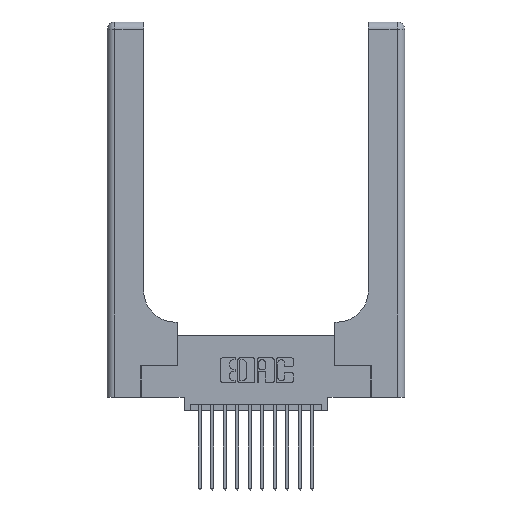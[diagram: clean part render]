
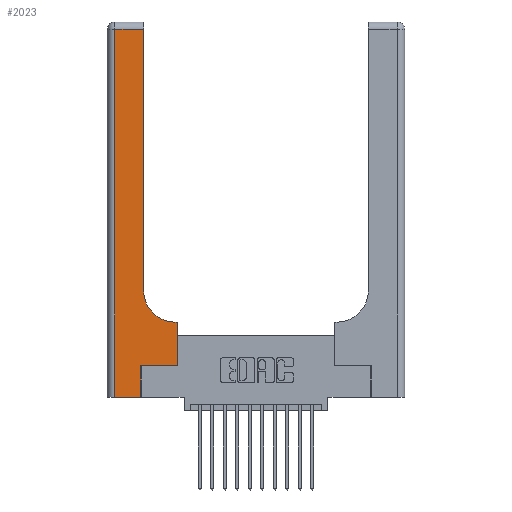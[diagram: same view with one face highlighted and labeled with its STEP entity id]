
A CAD part, top view. The second image highlights one B-rep face of the part: STEP entity #2023.
In plain terms, the highlighted planar face has unit normal (0, 0, 1).
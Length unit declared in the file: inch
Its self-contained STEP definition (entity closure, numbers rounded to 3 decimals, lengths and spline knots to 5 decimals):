
#156 = EDGE_CURVE ( 'NONE', #5343, #2314, #15026, .T. ) ;
#609 = VECTOR ( 'NONE', #10157, 39.37008 ) ;
#1039 = ORIENTED_EDGE ( 'NONE', *, *, #8074, .T. ) ;
#1229 = CARTESIAN_POINT ( 'NONE',  ( 0., 0., 0.37 ) ) ;
#1326 = ORIENTED_EDGE ( 'NONE', *, *, #4337, .T. ) ;
#1345 = ORIENTED_EDGE ( 'NONE', *, *, #6395, .T. ) ;
#1800 = AXIS2_PLACEMENT_3D ( 'NONE', #11598, #3505, #12896 ) ;
#1815 = VERTEX_POINT ( 'NONE', #11051 ) ;
#2023 = ADVANCED_FACE ( 'NONE', ( #11741 ), #4346, .F. ) ;
#2142 = ORIENTED_EDGE ( 'NONE', *, *, #12848, .T. ) ;
#2314 = VERTEX_POINT ( 'NONE', #16794 ) ;
#2365 = EDGE_CURVE ( 'NONE', #8949, #6291, #6749, .T. ) ;
#3494 = ORIENTED_EDGE ( 'NONE', *, *, #2365, .T. ) ;
#3505 = DIRECTION ( 'NONE',  ( 0., 0., -1. ) ) ;
#3654 = ORIENTED_EDGE ( 'NONE', *, *, #15591, .T. ) ;
#3823 = ORIENTED_EDGE ( 'NONE', *, *, #156, .T. ) ;
#4166 = DIRECTION ( 'NONE',  ( -1., 0., 0. ) ) ;
#4229 = DIRECTION ( 'NONE',  ( 0., 0., -1. ) ) ;
#4324 = CARTESIAN_POINT ( 'NONE',  ( 0., 3., 0.37 ) ) ;
#4337 = EDGE_CURVE ( 'NONE', #1815, #8949, #7239, .T. ) ;
#4341 = ORIENTED_EDGE ( 'NONE', *, *, #17361, .T. ) ;
#4346 = PLANE ( 'NONE',  #6728 ) ;
#4619 = CARTESIAN_POINT ( 'NONE',  ( 0.2915, 2.94, 0.37 ) ) ;
#5343 = VERTEX_POINT ( 'NONE', #15884 ) ;
#5420 = EDGE_CURVE ( 'NONE', #13145, #1815, #6986, .T. ) ;
#5740 = VERTEX_POINT ( 'NONE', #4619 ) ;
#5950 = CARTESIAN_POINT ( 'NONE',  ( 0.2915, 3., 0.37 ) ) ;
#5959 = VECTOR ( 'NONE', #12697, 39.37008 ) ;
#6291 = VERTEX_POINT ( 'NONE', #8607 ) ;
#6395 = EDGE_CURVE ( 'NONE', #7417, #13145, #7191, .T. ) ;
#6728 = AXIS2_PLACEMENT_3D ( 'NONE', #4324, #4229, #4166 ) ;
#6749 = LINE ( 'NONE', #14400, #10305 ) ;
#6913 = LINE ( 'NONE', #5950, #13512 ) ;
#6986 = LINE ( 'NONE', #10809, #17025 ) ;
#7191 = LINE ( 'NONE', #8815, #9913 ) ;
#7239 = LINE ( 'NONE', #11412, #5959 ) ;
#7324 = DIRECTION ( 'NONE',  ( 0., 1., 0. ) ) ;
#7353 = DIRECTION ( 'NONE',  ( -1., 0., 0. ) ) ;
#7417 = VERTEX_POINT ( 'NONE', #10851 ) ;
#8074 = EDGE_CURVE ( 'NONE', #5740, #5343, #14733, .T. ) ;
#8607 = CARTESIAN_POINT ( 'NONE',  ( 0.5415, 0.6, 0.37 ) ) ;
#8815 = CARTESIAN_POINT ( 'NONE',  ( 0.269, 0., 0.37 ) ) ;
#8949 = VERTEX_POINT ( 'NONE', #9300 ) ;
#9300 = CARTESIAN_POINT ( 'NONE',  ( 0.5585, 0.6, 0.37 ) ) ;
#9540 = DIRECTION ( 'NONE',  ( 1., 0., 0. ) ) ;
#9913 = VECTOR ( 'NONE', #16630, 39.37008 ) ;
#10157 = DIRECTION ( 'NONE',  ( 0., -1., 0. ) ) ;
#10181 = CARTESIAN_POINT ( 'NONE',  ( 0.06, 3., 0.37 ) ) ;
#10305 = VECTOR ( 'NONE', #14645, 39.37008 ) ;
#10323 = ORIENTED_EDGE ( 'NONE', *, *, #5420, .T. ) ;
#10809 = CARTESIAN_POINT ( 'NONE',  ( 0.269, 0.25, 0.37 ) ) ;
#10851 = CARTESIAN_POINT ( 'NONE',  ( 0.269, 0., 0.37 ) ) ;
#10952 = VERTEX_POINT ( 'NONE', #11157 ) ;
#11051 = CARTESIAN_POINT ( 'NONE',  ( 0.5585, 0.25, 0.37 ) ) ;
#11157 = CARTESIAN_POINT ( 'NONE',  ( 0.2915, 0.85, 0.37 ) ) ;
#11294 = CIRCLE ( 'NONE', #1800, 0.25 ) ;
#11412 = CARTESIAN_POINT ( 'NONE',  ( 0.5585, 0.25, 0.37 ) ) ;
#11598 = CARTESIAN_POINT ( 'NONE',  ( 0.5415, 0.85, 0.37 ) ) ;
#11741 = FACE_OUTER_BOUND ( 'NONE', #14162, .T. ) ;
#12697 = DIRECTION ( 'NONE',  ( 0., 1., 0. ) ) ;
#12848 = EDGE_CURVE ( 'NONE', #2314, #7417, #14410, .T. ) ;
#12896 = DIRECTION ( 'NONE',  ( 1., 0., 0. ) ) ;
#13145 = VERTEX_POINT ( 'NONE', #16583 ) ;
#13432 = DIRECTION ( 'NONE',  ( 1., 0., 0. ) ) ;
#13512 = VECTOR ( 'NONE', #7324, 39.37008 ) ;
#14162 = EDGE_LOOP ( 'NONE', ( #3654, #1039, #3823, #2142, #1345, #10323, #1326, #3494, #4341 ) ) ;
#14400 = CARTESIAN_POINT ( 'NONE',  ( 0.2915, 0.6, 0.37 ) ) ;
#14410 = LINE ( 'NONE', #1229, #17450 ) ;
#14645 = DIRECTION ( 'NONE',  ( -1., 0., 0. ) ) ;
#14733 = LINE ( 'NONE', #16509, #17374 ) ;
#15026 = LINE ( 'NONE', #10181, #609 ) ;
#15591 = EDGE_CURVE ( 'NONE', #10952, #5740, #6913, .T. ) ;
#15884 = CARTESIAN_POINT ( 'NONE',  ( 0.06, 2.94, 0.37 ) ) ;
#16509 = CARTESIAN_POINT ( 'NONE',  ( 0., 2.94, 0.37 ) ) ;
#16583 = CARTESIAN_POINT ( 'NONE',  ( 0.269, 0.25, 0.37 ) ) ;
#16630 = DIRECTION ( 'NONE',  ( 0., 1., 0. ) ) ;
#16794 = CARTESIAN_POINT ( 'NONE',  ( 0.06, 0., 0.37 ) ) ;
#17025 = VECTOR ( 'NONE', #13432, 39.37008 ) ;
#17361 = EDGE_CURVE ( 'NONE', #6291, #10952, #11294, .T. ) ;
#17374 = VECTOR ( 'NONE', #7353, 39.37008 ) ;
#17450 = VECTOR ( 'NONE', #9540, 39.37008 ) ;
